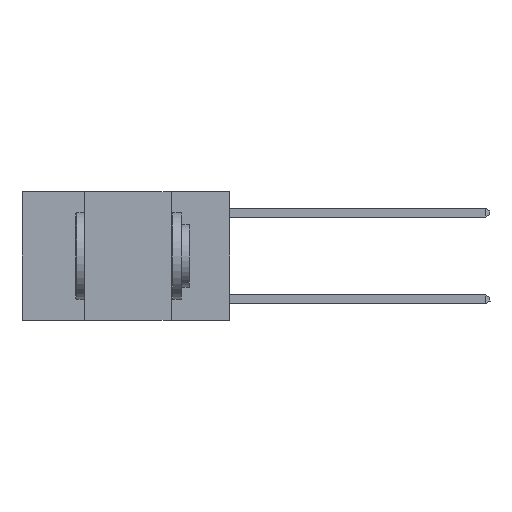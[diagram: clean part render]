
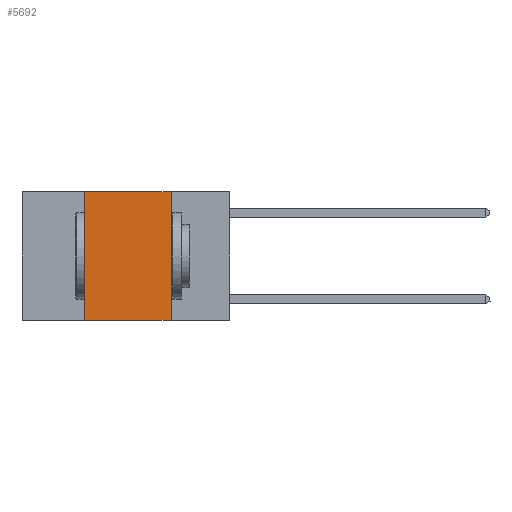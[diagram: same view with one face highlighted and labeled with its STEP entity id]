
A CAD part, left-side view. The second image highlights one B-rep face of the part: STEP entity #5692.
In plain terms, the highlighted planar face has unit normal (-1, 0, 0).
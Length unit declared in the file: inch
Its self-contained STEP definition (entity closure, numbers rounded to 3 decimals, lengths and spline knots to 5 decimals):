
#121 = LINE ( 'NONE', #13827, #5894 ) ;
#200 = VECTOR ( 'NONE', #9412, 39.37008 ) ;
#204 = EDGE_LOOP ( 'NONE', ( #467, #3643, #6512, #6552 ) ) ;
#413 = CARTESIAN_POINT ( 'NONE',  ( 0., 0.6, 0. ) ) ;
#467 = ORIENTED_EDGE ( 'NONE', *, *, #6251, .F. ) ;
#1145 = CARTESIAN_POINT ( 'NONE',  ( 0., 0.17, -0.37 ) ) ;
#1178 = LINE ( 'NONE', #2053, #9769 ) ;
#1312 = LINE ( 'NONE', #11145, #7059 ) ;
#1774 = DIRECTION ( 'NONE',  ( 0., -1., 0. ) ) ;
#2053 = CARTESIAN_POINT ( 'NONE',  ( 0., 0.17, 0. ) ) ;
#2905 = PLANE ( 'NONE',  #12645 ) ;
#3643 = ORIENTED_EDGE ( 'NONE', *, *, #11346, .F. ) ;
#4001 = LINE ( 'NONE', #413, #200 ) ;
#4076 = DIRECTION ( 'NONE',  ( 1., 0., 0. ) ) ;
#5054 = FACE_OUTER_BOUND ( 'NONE', #204, .T. ) ;
#5078 = VERTEX_POINT ( 'NONE', #13914 ) ;
#5692 = ADVANCED_FACE ( 'NONE', ( #5054 ), #2905, .F. ) ;
#5894 = VECTOR ( 'NONE', #1774, 39.37008 ) ;
#6251 = EDGE_CURVE ( 'NONE', #12092, #6420, #1178, .T. ) ;
#6420 = VERTEX_POINT ( 'NONE', #1145 ) ;
#6458 = VERTEX_POINT ( 'NONE', #9065 ) ;
#6512 = ORIENTED_EDGE ( 'NONE', *, *, #8179, .F. ) ;
#6552 = ORIENTED_EDGE ( 'NONE', *, *, #6910, .T. ) ;
#6706 = DIRECTION ( 'NONE',  ( 0., 0., -1. ) ) ;
#6910 = EDGE_CURVE ( 'NONE', #5078, #6420, #121, .T. ) ;
#7059 = VECTOR ( 'NONE', #12217, 39.37008 ) ;
#7419 = CARTESIAN_POINT ( 'NONE',  ( 0., 0.6, 0. ) ) ;
#8179 = EDGE_CURVE ( 'NONE', #5078, #6458, #1312, .T. ) ;
#9065 = CARTESIAN_POINT ( 'NONE',  ( 0., 0.42, 0. ) ) ;
#9412 = DIRECTION ( 'NONE',  ( 0., -1., 0. ) ) ;
#9769 = VECTOR ( 'NONE', #6706, 39.37008 ) ;
#11145 = CARTESIAN_POINT ( 'NONE',  ( 0., 0.42, 0. ) ) ;
#11346 = EDGE_CURVE ( 'NONE', #6458, #12092, #4001, .T. ) ;
#11698 = DIRECTION ( 'NONE',  ( 0., 0., -1. ) ) ;
#12092 = VERTEX_POINT ( 'NONE', #12462 ) ;
#12217 = DIRECTION ( 'NONE',  ( 0., 0., 1. ) ) ;
#12462 = CARTESIAN_POINT ( 'NONE',  ( 0., 0.17, 0. ) ) ;
#12645 = AXIS2_PLACEMENT_3D ( 'NONE', #7419, #4076, #11698 ) ;
#13827 = CARTESIAN_POINT ( 'NONE',  ( 0., 0.6, -0.37 ) ) ;
#13914 = CARTESIAN_POINT ( 'NONE',  ( 0., 0.42, -0.37 ) ) ;
